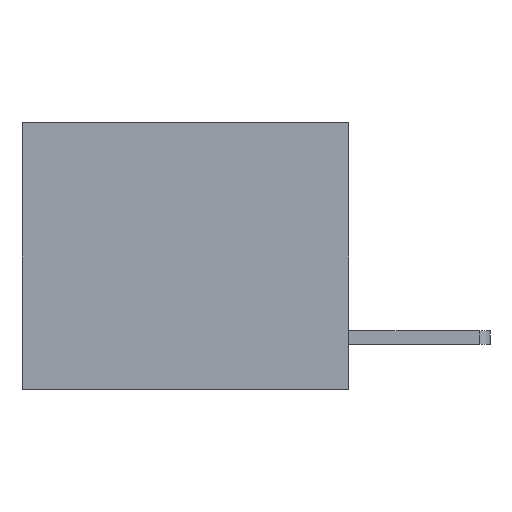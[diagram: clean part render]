
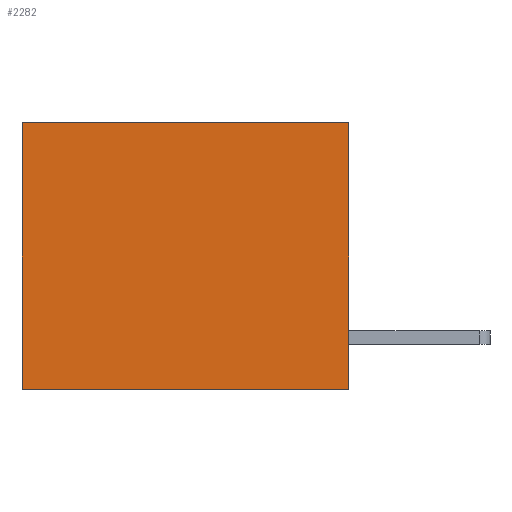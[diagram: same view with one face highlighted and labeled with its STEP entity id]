
A CAD part, left-side view. The second image highlights one B-rep face of the part: STEP entity #2282.
In plain terms, the highlighted planar face has unit normal (-1, 0, 0).
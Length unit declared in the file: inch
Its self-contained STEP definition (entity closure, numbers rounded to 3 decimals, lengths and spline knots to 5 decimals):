
#69 = VERTEX_POINT ( 'NONE', #145 ) ;
#145 = CARTESIAN_POINT ( 'NONE',  ( 0.3165, 0.6, -0.49 ) ) ;
#723 = VERTEX_POINT ( 'NONE', #2934 ) ;
#737 = VECTOR ( 'NONE', #1321, 39.37008 ) ;
#880 = DIRECTION ( 'NONE',  ( 0., 1., 0. ) ) ;
#911 = ORIENTED_EDGE ( 'NONE', *, *, #6213, .F. ) ;
#1126 = CARTESIAN_POINT ( 'NONE',  ( 0.3165, 0., 0. ) ) ;
#1291 = VECTOR ( 'NONE', #6004, 39.37008 ) ;
#1321 = DIRECTION ( 'NONE',  ( 0., 0., -1. ) ) ;
#1418 = CARTESIAN_POINT ( 'NONE',  ( 0.3165, 0., -0.49 ) ) ;
#1573 = VERTEX_POINT ( 'NONE', #1418 ) ;
#2282 = ADVANCED_FACE ( 'NONE', ( #7637 ), #7661, .F. ) ;
#2626 = EDGE_LOOP ( 'NONE', ( #5202, #3695, #911, #4473 ) ) ;
#2740 = EDGE_CURVE ( 'NONE', #1573, #69, #5774, .T. ) ;
#2934 = CARTESIAN_POINT ( 'NONE',  ( 0.3165, 0.6, 0. ) ) ;
#3332 = CARTESIAN_POINT ( 'NONE',  ( 0.3165, 0., -0.49 ) ) ;
#3358 = CARTESIAN_POINT ( 'NONE',  ( 0.3165, 0., -0.49 ) ) ;
#3695 = ORIENTED_EDGE ( 'NONE', *, *, #2740, .F. ) ;
#3851 = DIRECTION ( 'NONE',  ( 0., 0., -1. ) ) ;
#4315 = EDGE_CURVE ( 'NONE', #723, #69, #5654, .T. ) ;
#4473 = ORIENTED_EDGE ( 'NONE', *, *, #6415, .T. ) ;
#4584 = LINE ( 'NONE', #3358, #7961 ) ;
#4778 = CARTESIAN_POINT ( 'NONE',  ( 0.3165, 0., 0. ) ) ;
#4986 = VERTEX_POINT ( 'NONE', #4778 ) ;
#5202 = ORIENTED_EDGE ( 'NONE', *, *, #4315, .T. ) ;
#5381 = CARTESIAN_POINT ( 'NONE',  ( 0.3165, 0., -0.49 ) ) ;
#5411 = DIRECTION ( 'NONE',  ( 0., 0., -1. ) ) ;
#5654 = LINE ( 'NONE', #6263, #737 ) ;
#5774 = LINE ( 'NONE', #3332, #6819 ) ;
#6004 = DIRECTION ( 'NONE',  ( 0., 1., 0. ) ) ;
#6213 = EDGE_CURVE ( 'NONE', #4986, #1573, #4584, .T. ) ;
#6263 = CARTESIAN_POINT ( 'NONE',  ( 0.3165, 0.6, -0.49 ) ) ;
#6415 = EDGE_CURVE ( 'NONE', #4986, #723, #7762, .T. ) ;
#6548 = AXIS2_PLACEMENT_3D ( 'NONE', #5381, #7779, #5411 ) ;
#6819 = VECTOR ( 'NONE', #880, 39.37008 ) ;
#7637 = FACE_OUTER_BOUND ( 'NONE', #2626, .T. ) ;
#7661 = PLANE ( 'NONE',  #6548 ) ;
#7762 = LINE ( 'NONE', #1126, #1291 ) ;
#7779 = DIRECTION ( 'NONE',  ( 1., 0., 0. ) ) ;
#7961 = VECTOR ( 'NONE', #3851, 39.37008 ) ;
